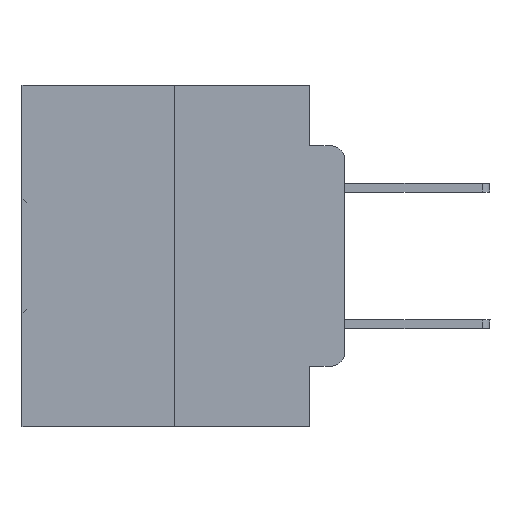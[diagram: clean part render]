
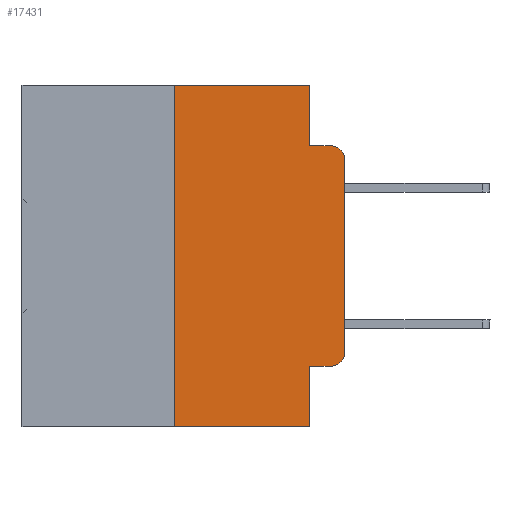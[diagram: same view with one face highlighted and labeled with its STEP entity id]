
A CAD part, left-side view. The second image highlights one B-rep face of the part: STEP entity #17431.
In plain terms, the highlighted planar face has unit normal (-1, 0, 0).
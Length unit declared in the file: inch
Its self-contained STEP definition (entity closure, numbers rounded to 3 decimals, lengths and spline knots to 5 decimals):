
#405 = DIRECTION ( 'NONE',  ( 0., 0., -1. ) ) ;
#454 = CARTESIAN_POINT ( 'NONE',  ( 0., 0., -0.3915 ) ) ;
#597 = VECTOR ( 'NONE', #26012, 39.37008 ) ;
#1536 = CARTESIAN_POINT ( 'NONE',  ( 0., 0.02, -0.1085 ) ) ;
#1899 = LINE ( 'NONE', #22246, #17670 ) ;
#1996 = VERTEX_POINT ( 'NONE', #27354 ) ;
#2618 = CARTESIAN_POINT ( 'NONE',  ( 0., 0.02, -0.0885 ) ) ;
#2784 = ORIENTED_EDGE ( 'NONE', *, *, #19541, .F. ) ;
#2818 = CIRCLE ( 'NONE', #21781, 0.02 ) ;
#3108 = PLANE ( 'NONE',  #26873 ) ;
#3148 = CARTESIAN_POINT ( 'NONE',  ( 0., 0.25, 0. ) ) ;
#3470 = CARTESIAN_POINT ( 'NONE',  ( 0., 0.473, -0.5 ) ) ;
#3473 = CARTESIAN_POINT ( 'NONE',  ( 0., 0.051, -0.0885 ) ) ;
#3956 = CARTESIAN_POINT ( 'NONE',  ( 0., 0.051, -0.0885 ) ) ;
#5007 = DIRECTION ( 'NONE',  ( 1., 0., 0. ) ) ;
#5123 = CARTESIAN_POINT ( 'NONE',  ( 0., 0.25, -0.5 ) ) ;
#5671 = FACE_OUTER_BOUND ( 'NONE', #17406, .T. ) ;
#6806 = ORIENTED_EDGE ( 'NONE', *, *, #22020, .T. ) ;
#6968 = ORIENTED_EDGE ( 'NONE', *, *, #16390, .T. ) ;
#7528 = VERTEX_POINT ( 'NONE', #19707 ) ;
#8546 = DIRECTION ( 'NONE',  ( 0., 0., -1. ) ) ;
#10742 = ORIENTED_EDGE ( 'NONE', *, *, #29924, .T. ) ;
#10836 = ORIENTED_EDGE ( 'NONE', *, *, #22870, .F. ) ;
#11175 = LINE ( 'NONE', #14215, #31502 ) ;
#11272 = VECTOR ( 'NONE', #16046, 39.37008 ) ;
#12095 = LINE ( 'NONE', #3470, #22197 ) ;
#12918 = DIRECTION ( 'NONE',  ( 0., 0., -1. ) ) ;
#13053 = VERTEX_POINT ( 'NONE', #2618 ) ;
#13308 = CARTESIAN_POINT ( 'NONE',  ( 0., 0.051, -0.4115 ) ) ;
#13319 = LINE ( 'NONE', #23645, #21151 ) ;
#14215 = CARTESIAN_POINT ( 'NONE',  ( 0., 0.473, 0. ) ) ;
#14250 = ORIENTED_EDGE ( 'NONE', *, *, #18221, .T. ) ;
#14561 = VERTEX_POINT ( 'NONE', #15881 ) ;
#14965 = LINE ( 'NONE', #20391, #25818 ) ;
#15089 = VERTEX_POINT ( 'NONE', #3956 ) ;
#15426 = CARTESIAN_POINT ( 'NONE',  ( 0., 0.051, 0. ) ) ;
#15881 = CARTESIAN_POINT ( 'NONE',  ( 0., 0.02, -0.4115 ) ) ;
#15953 = CARTESIAN_POINT ( 'NONE',  ( 0., 0.02, -0.3915 ) ) ;
#16046 = DIRECTION ( 'NONE',  ( 0., -1., 0. ) ) ;
#16372 = LINE ( 'NONE', #3473, #11272 ) ;
#16390 = EDGE_CURVE ( 'NONE', #16628, #18130, #1899, .T. ) ;
#16628 = VERTEX_POINT ( 'NONE', #454 ) ;
#16809 = CARTESIAN_POINT ( 'NONE',  ( 0., 0., -0.1085 ) ) ;
#17406 = EDGE_LOOP ( 'NONE', ( #6968, #14250, #23311, #26784, #28846, #2784, #6806, #10836, #10742, #21144 ) ) ;
#17431 = ADVANCED_FACE ( 'NONE', ( #5671 ), #3108, .F. ) ;
#17497 = EDGE_CURVE ( 'NONE', #21288, #15089, #19408, .T. ) ;
#17670 = VECTOR ( 'NONE', #27842, 39.37008 ) ;
#18130 = VERTEX_POINT ( 'NONE', #16809 ) ;
#18221 = EDGE_CURVE ( 'NONE', #18130, #13053, #27945, .T. ) ;
#18664 = DIRECTION ( 'NONE',  ( -1., 0., 0. ) ) ;
#19259 = VECTOR ( 'NONE', #8546, 39.37008 ) ;
#19408 = LINE ( 'NONE', #32090, #19259 ) ;
#19477 = DIRECTION ( 'NONE',  ( 0., -1., 0. ) ) ;
#19528 = DIRECTION ( 'NONE',  ( -1., 0., 0. ) ) ;
#19541 = EDGE_CURVE ( 'NONE', #30895, #24224, #14965, .T. ) ;
#19707 = CARTESIAN_POINT ( 'NONE',  ( 0., 0.051, -0.4115 ) ) ;
#19732 = DIRECTION ( 'NONE',  ( 0., -1., 0. ) ) ;
#20162 = EDGE_CURVE ( 'NONE', #15089, #13053, #16372, .T. ) ;
#20391 = CARTESIAN_POINT ( 'NONE',  ( 0., 0.25, 0. ) ) ;
#21144 = ORIENTED_EDGE ( 'NONE', *, *, #30947, .T. ) ;
#21151 = VECTOR ( 'NONE', #405, 39.37008 ) ;
#21288 = VERTEX_POINT ( 'NONE', #15426 ) ;
#21781 = AXIS2_PLACEMENT_3D ( 'NONE', #15953, #18664, #12918 ) ;
#22020 = EDGE_CURVE ( 'NONE', #30895, #1996, #12095, .T. ) ;
#22197 = VECTOR ( 'NONE', #19732, 39.37008 ) ;
#22246 = CARTESIAN_POINT ( 'NONE',  ( 0., 0., 0. ) ) ;
#22870 = EDGE_CURVE ( 'NONE', #7528, #1996, #13319, .T. ) ;
#23311 = ORIENTED_EDGE ( 'NONE', *, *, #20162, .F. ) ;
#23632 = LINE ( 'NONE', #13308, #597 ) ;
#23645 = CARTESIAN_POINT ( 'NONE',  ( 0., 0.051, 0. ) ) ;
#24137 = AXIS2_PLACEMENT_3D ( 'NONE', #1536, #19528, #29842 ) ;
#24224 = VERTEX_POINT ( 'NONE', #3148 ) ;
#25126 = DIRECTION ( 'NONE',  ( 0., 0., 1. ) ) ;
#25818 = VECTOR ( 'NONE', #25126, 39.37008 ) ;
#25999 = CARTESIAN_POINT ( 'NONE',  ( 0., 0.473, 0. ) ) ;
#26012 = DIRECTION ( 'NONE',  ( 0., -1., 0. ) ) ;
#26784 = ORIENTED_EDGE ( 'NONE', *, *, #17497, .F. ) ;
#26873 = AXIS2_PLACEMENT_3D ( 'NONE', #25999, #5007, #31404 ) ;
#27354 = CARTESIAN_POINT ( 'NONE',  ( 0., 0.051, -0.5 ) ) ;
#27842 = DIRECTION ( 'NONE',  ( 0., 0., 1. ) ) ;
#27945 = CIRCLE ( 'NONE', #24137, 0.02 ) ;
#28846 = ORIENTED_EDGE ( 'NONE', *, *, #32812, .F. ) ;
#29842 = DIRECTION ( 'NONE',  ( 0., 0., -1. ) ) ;
#29924 = EDGE_CURVE ( 'NONE', #7528, #14561, #23632, .T. ) ;
#30895 = VERTEX_POINT ( 'NONE', #5123 ) ;
#30947 = EDGE_CURVE ( 'NONE', #14561, #16628, #2818, .T. ) ;
#31404 = DIRECTION ( 'NONE',  ( 0., 0., -1. ) ) ;
#31502 = VECTOR ( 'NONE', #19477, 39.37008 ) ;
#32090 = CARTESIAN_POINT ( 'NONE',  ( 0., 0.051, 0. ) ) ;
#32812 = EDGE_CURVE ( 'NONE', #24224, #21288, #11175, .T. ) ;
